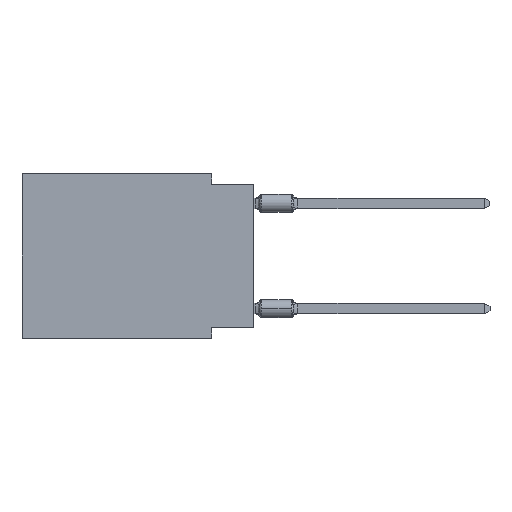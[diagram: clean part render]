
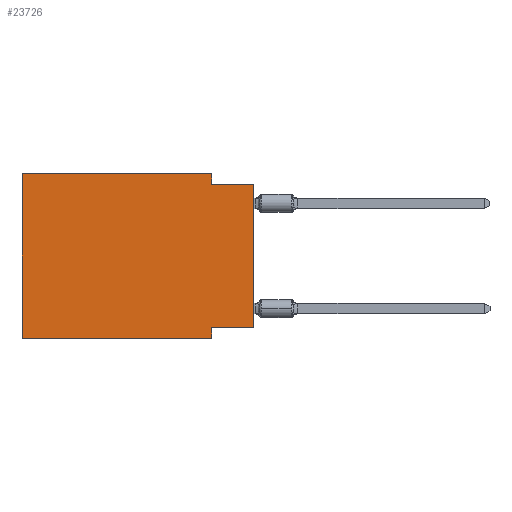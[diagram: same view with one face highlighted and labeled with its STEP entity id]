
A CAD part, left-side view. The second image highlights one B-rep face of the part: STEP entity #23726.
In plain terms, the highlighted planar face has unit normal (-1, 0, 0).
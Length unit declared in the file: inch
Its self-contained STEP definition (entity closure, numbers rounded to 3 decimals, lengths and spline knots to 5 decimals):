
#580 = DIRECTION ( 'NONE',  ( 0., 1., 0. ) ) ;
#988 = ORIENTED_EDGE ( 'NONE', *, *, #7503, .F. ) ;
#1248 = CARTESIAN_POINT ( 'NONE',  ( 0., 0.1, -0.39 ) ) ;
#1316 = VECTOR ( 'NONE', #1715, 39.37008 ) ;
#1372 = CARTESIAN_POINT ( 'NONE',  ( 0., 0.1, 0. ) ) ;
#1715 = DIRECTION ( 'NONE',  ( 0., -1., 0. ) ) ;
#1810 = VERTEX_POINT ( 'NONE', #8209 ) ;
#2192 = VERTEX_POINT ( 'NONE', #7754 ) ;
#2214 = CARTESIAN_POINT ( 'NONE',  ( 0., 0., 0. ) ) ;
#2393 = LINE ( 'NONE', #20522, #2962 ) ;
#2629 = CARTESIAN_POINT ( 'NONE',  ( 0., 0.55, -0.39 ) ) ;
#2663 = VERTEX_POINT ( 'NONE', #8376 ) ;
#2962 = VECTOR ( 'NONE', #580, 39.37008 ) ;
#3703 = DIRECTION ( 'NONE',  ( 0., 0., -1. ) ) ;
#3772 = LINE ( 'NONE', #2214, #9446 ) ;
#4022 = CARTESIAN_POINT ( 'NONE',  ( 0., 0.1, -0.025 ) ) ;
#4057 = VERTEX_POINT ( 'NONE', #4022 ) ;
#4118 = DIRECTION ( 'NONE',  ( 0., 0., 1. ) ) ;
#4173 = DIRECTION ( 'NONE',  ( 0., -1., 0. ) ) ;
#4734 = EDGE_CURVE ( 'NONE', #9552, #1810, #22633, .T. ) ;
#5611 = ORIENTED_EDGE ( 'NONE', *, *, #25328, .T. ) ;
#5636 = PLANE ( 'NONE',  #14010 ) ;
#6666 = ORIENTED_EDGE ( 'NONE', *, *, #21583, .F. ) ;
#7022 = CARTESIAN_POINT ( 'NONE',  ( 0., 0.55, 0. ) ) ;
#7341 = DIRECTION ( 'NONE',  ( 0., 0., -1. ) ) ;
#7367 = LINE ( 'NONE', #21607, #7774 ) ;
#7503 = EDGE_CURVE ( 'NONE', #4057, #13990, #7367, .T. ) ;
#7754 = CARTESIAN_POINT ( 'NONE',  ( 0., 0., -0.365 ) ) ;
#7774 = VECTOR ( 'NONE', #23541, 39.37008 ) ;
#8209 = CARTESIAN_POINT ( 'NONE',  ( 0., 0.1, -0.39 ) ) ;
#8376 = CARTESIAN_POINT ( 'NONE',  ( 0., 0.1, 0. ) ) ;
#8662 = ORIENTED_EDGE ( 'NONE', *, *, #9555, .T. ) ;
#8793 = ORIENTED_EDGE ( 'NONE', *, *, #4734, .F. ) ;
#9446 = VECTOR ( 'NONE', #23712, 39.37008 ) ;
#9552 = VERTEX_POINT ( 'NONE', #21654 ) ;
#9555 = EDGE_CURVE ( 'NONE', #2192, #13990, #3772, .T. ) ;
#11696 = LINE ( 'NONE', #25408, #23361 ) ;
#11846 = VECTOR ( 'NONE', #3703, 39.37008 ) ;
#11865 = FACE_OUTER_BOUND ( 'NONE', #20588, .T. ) ;
#12843 = CARTESIAN_POINT ( 'NONE',  ( 0., 0., -0.025 ) ) ;
#13475 = VECTOR ( 'NONE', #7341, 39.37008 ) ;
#13513 = LINE ( 'NONE', #17780, #1316 ) ;
#13542 = CARTESIAN_POINT ( 'NONE',  ( 0., 0.55, 0. ) ) ;
#13973 = CARTESIAN_POINT ( 'NONE',  ( 0., 0.55, 0. ) ) ;
#13990 = VERTEX_POINT ( 'NONE', #12843 ) ;
#14010 = AXIS2_PLACEMENT_3D ( 'NONE', #13542, #25433, #23886 ) ;
#15231 = LINE ( 'NONE', #1372, #11846 ) ;
#17780 = CARTESIAN_POINT ( 'NONE',  ( 0., 0.55, -0.39 ) ) ;
#17784 = VERTEX_POINT ( 'NONE', #2629 ) ;
#17898 = VERTEX_POINT ( 'NONE', #7022 ) ;
#18911 = VECTOR ( 'NONE', #4118, 39.37008 ) ;
#19332 = ORIENTED_EDGE ( 'NONE', *, *, #20134, .F. ) ;
#19477 = EDGE_CURVE ( 'NONE', #17898, #2663, #11696, .T. ) ;
#19655 = ORIENTED_EDGE ( 'NONE', *, *, #19477, .F. ) ;
#20134 = EDGE_CURVE ( 'NONE', #2663, #4057, #15231, .T. ) ;
#20522 = CARTESIAN_POINT ( 'NONE',  ( 0., 0., -0.365 ) ) ;
#20588 = EDGE_LOOP ( 'NONE', ( #8662, #988, #19332, #19655, #6666, #5611, #8793, #21457 ) ) ;
#21457 = ORIENTED_EDGE ( 'NONE', *, *, #25003, .F. ) ;
#21583 = EDGE_CURVE ( 'NONE', #17784, #17898, #25221, .T. ) ;
#21607 = CARTESIAN_POINT ( 'NONE',  ( 0., 0., -0.025 ) ) ;
#21654 = CARTESIAN_POINT ( 'NONE',  ( 0., 0.1, -0.365 ) ) ;
#22633 = LINE ( 'NONE', #1248, #13475 ) ;
#23361 = VECTOR ( 'NONE', #4173, 39.37008 ) ;
#23541 = DIRECTION ( 'NONE',  ( 0., -1., 0. ) ) ;
#23712 = DIRECTION ( 'NONE',  ( 0., 0., 1. ) ) ;
#23726 = ADVANCED_FACE ( 'NONE', ( #11865 ), #5636, .F. ) ;
#23886 = DIRECTION ( 'NONE',  ( 0., 0., -1. ) ) ;
#25003 = EDGE_CURVE ( 'NONE', #2192, #9552, #2393, .T. ) ;
#25221 = LINE ( 'NONE', #13973, #18911 ) ;
#25328 = EDGE_CURVE ( 'NONE', #17784, #1810, #13513, .T. ) ;
#25408 = CARTESIAN_POINT ( 'NONE',  ( 0., 0.55, 0. ) ) ;
#25433 = DIRECTION ( 'NONE',  ( 1., 0., 0. ) ) ;
